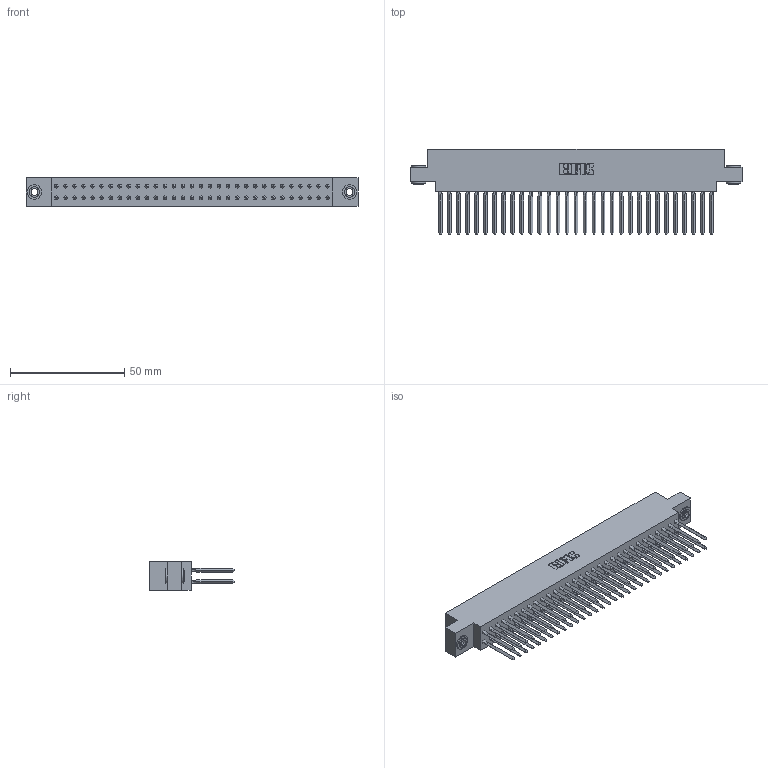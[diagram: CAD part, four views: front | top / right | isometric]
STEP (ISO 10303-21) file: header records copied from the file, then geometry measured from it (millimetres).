
FILE_DESCRIPTION (( 'STEP AP203' ), '1' );
FILE_NAME ('317-062-542-803.STEP', '2020-02-28T05:29:12', ( '' ), ( '' ), 'SwSTEP 2.0', 'SolidWorks 2016', '' );
FILE_SCHEMA (( 'CONFIG_CONTROL_DESIGN' ));
Length unit declared in the file: inch
Products named in the file (4): 317 Part_.156 Dia - TH; 317-290-003_542; 317-062-542-803; 345-250-002_345-250-002-102
Assembly tree (65 placements, depth 2):
  317-062-542-803
    317 Part_.156 Dia - TH
    317-290-003_542  x62
    345-250-002_345-250-002-102  x2
Bounding box: 145.54 x 37.34 x 12.7 mm (x, y, z)
Volume: 23503.8 mm3; surface area: 32547.5 mm2
Topology: 65 solids, 65 shells, 3674 faces, 10271 edges, 6554 vertices
Faces by surface type: plane 2920, cylinder 498, bspline 248, cone 8
Entity records: 46012 total; most frequent: CARTESIAN_POINT 8244, ORIENTED_EDGE 7900, DIRECTION 6704, EDGE_CURVE 3950, VECTOR 3756, LINE 3756, VERTEX_POINT 2626, AXIS2_PLACEMENT_3D 1474
